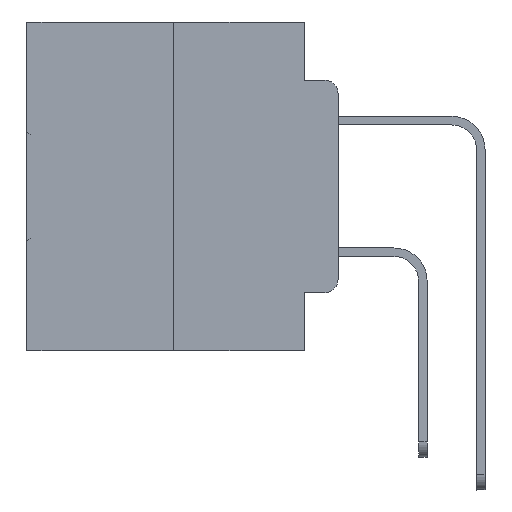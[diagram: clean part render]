
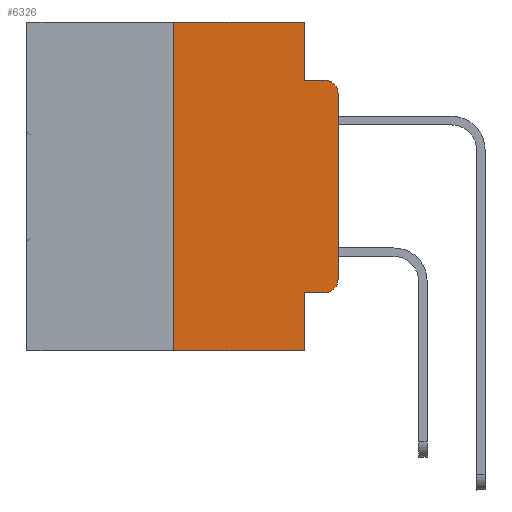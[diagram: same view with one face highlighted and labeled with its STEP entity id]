
A CAD part, left-side view. The second image highlights one B-rep face of the part: STEP entity #6326.
In plain terms, the highlighted planar face has unit normal (-1, 0, 0).
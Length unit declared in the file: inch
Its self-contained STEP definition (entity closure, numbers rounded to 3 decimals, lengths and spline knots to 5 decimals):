
#395 = CARTESIAN_POINT ( 'NONE',  ( 0., 0.051, -0.4115 ) ) ;
#605 = DIRECTION ( 'NONE',  ( 0., -1., 0. ) ) ;
#1468 = CARTESIAN_POINT ( 'NONE',  ( 0., 0.051, 0. ) ) ;
#1921 = CARTESIAN_POINT ( 'NONE',  ( 0., 0.473, 0. ) ) ;
#2920 = ORIENTED_EDGE ( 'NONE', *, *, #32133, .T. ) ;
#3748 = VERTEX_POINT ( 'NONE', #19978 ) ;
#4130 = ORIENTED_EDGE ( 'NONE', *, *, #6447, .T. ) ;
#4686 = FACE_OUTER_BOUND ( 'NONE', #32438, .T. ) ;
#4892 = LINE ( 'NONE', #25082, #20230 ) ;
#4902 = DIRECTION ( 'NONE',  ( 0., -1., 0. ) ) ;
#5497 = VECTOR ( 'NONE', #4902, 39.37008 ) ;
#5581 = VECTOR ( 'NONE', #5647, 39.37008 ) ;
#5647 = DIRECTION ( 'NONE',  ( 0., 0., 1. ) ) ;
#5932 = LINE ( 'NONE', #33000, #19574 ) ;
#6000 = EDGE_CURVE ( 'NONE', #9498, #12950, #12390, .T. ) ;
#6326 = ADVANCED_FACE ( 'NONE', ( #4686 ), #10875, .F. ) ;
#6447 = EDGE_CURVE ( 'NONE', #14063, #12950, #5932, .T. ) ;
#6592 = CARTESIAN_POINT ( 'NONE',  ( 0., 0.02, -0.1085 ) ) ;
#6674 = CARTESIAN_POINT ( 'NONE',  ( 0., 0.25, 0. ) ) ;
#6714 = VECTOR ( 'NONE', #28657, 39.37008 ) ;
#7404 = VECTOR ( 'NONE', #19513, 39.37008 ) ;
#7752 = AXIS2_PLACEMENT_3D ( 'NONE', #6592, #25586, #9332 ) ;
#7899 = EDGE_CURVE ( 'NONE', #23251, #21904, #24966, .T. ) ;
#8251 = DIRECTION ( 'NONE',  ( 0., 0., -1. ) ) ;
#9046 = EDGE_CURVE ( 'NONE', #9549, #3748, #10031, .T. ) ;
#9076 = ORIENTED_EDGE ( 'NONE', *, *, #33514, .F. ) ;
#9156 = CARTESIAN_POINT ( 'NONE',  ( 0., 0.051, -0.0885 ) ) ;
#9332 = DIRECTION ( 'NONE',  ( 0., 0., -1. ) ) ;
#9498 = VERTEX_POINT ( 'NONE', #395 ) ;
#9549 = VERTEX_POINT ( 'NONE', #22388 ) ;
#10031 = CIRCLE ( 'NONE', #12363, 0.02 ) ;
#10875 = PLANE ( 'NONE',  #23406 ) ;
#11300 = ORIENTED_EDGE ( 'NONE', *, *, #7899, .T. ) ;
#11799 = ORIENTED_EDGE ( 'NONE', *, *, #14082, .F. ) ;
#12113 = DIRECTION ( 'NONE',  ( -1., 0., 0. ) ) ;
#12363 = AXIS2_PLACEMENT_3D ( 'NONE', #28296, #12113, #30946 ) ;
#12390 = LINE ( 'NONE', #1468, #25947 ) ;
#12442 = DIRECTION ( 'NONE',  ( 0., 0., -1. ) ) ;
#12760 = LINE ( 'NONE', #1921, #5497 ) ;
#12950 = VERTEX_POINT ( 'NONE', #31614 ) ;
#13014 = EDGE_CURVE ( 'NONE', #30397, #27172, #12760, .T. ) ;
#13642 = VECTOR ( 'NONE', #22838, 39.37008 ) ;
#13964 = LINE ( 'NONE', #28777, #6714 ) ;
#14063 = VERTEX_POINT ( 'NONE', #20664 ) ;
#14082 = EDGE_CURVE ( 'NONE', #27130, #21904, #13964, .T. ) ;
#14679 = LINE ( 'NONE', #19395, #7404 ) ;
#15423 = ORIENTED_EDGE ( 'NONE', *, *, #6000, .F. ) ;
#15565 = EDGE_CURVE ( 'NONE', #27172, #27130, #4892, .T. ) ;
#16531 = CARTESIAN_POINT ( 'NONE',  ( 0., 0.25, 0. ) ) ;
#19069 = CARTESIAN_POINT ( 'NONE',  ( 0., 0.473, 0. ) ) ;
#19395 = CARTESIAN_POINT ( 'NONE',  ( 0., 0.051, -0.4115 ) ) ;
#19513 = DIRECTION ( 'NONE',  ( 0., -1., 0. ) ) ;
#19574 = VECTOR ( 'NONE', #605, 39.37008 ) ;
#19978 = CARTESIAN_POINT ( 'NONE',  ( 0., 0., -0.3915 ) ) ;
#20122 = CARTESIAN_POINT ( 'NONE',  ( 0., 0., 0. ) ) ;
#20230 = VECTOR ( 'NONE', #27755, 39.37008 ) ;
#20664 = CARTESIAN_POINT ( 'NONE',  ( 0., 0.25, -0.5 ) ) ;
#21017 = ORIENTED_EDGE ( 'NONE', *, *, #9046, .T. ) ;
#21904 = VERTEX_POINT ( 'NONE', #29065 ) ;
#22388 = CARTESIAN_POINT ( 'NONE',  ( 0., 0.02, -0.4115 ) ) ;
#22838 = DIRECTION ( 'NONE',  ( 0., 0., 1. ) ) ;
#23251 = VERTEX_POINT ( 'NONE', #29214 ) ;
#23406 = AXIS2_PLACEMENT_3D ( 'NONE', #19069, #24498, #8251 ) ;
#23587 = ORIENTED_EDGE ( 'NONE', *, *, #15565, .F. ) ;
#23698 = ORIENTED_EDGE ( 'NONE', *, *, #13014, .F. ) ;
#24498 = DIRECTION ( 'NONE',  ( 1., 0., 0. ) ) ;
#24714 = ORIENTED_EDGE ( 'NONE', *, *, #34378, .T. ) ;
#24966 = CIRCLE ( 'NONE', #7752, 0.02 ) ;
#25082 = CARTESIAN_POINT ( 'NONE',  ( 0., 0.051, 0. ) ) ;
#25586 = DIRECTION ( 'NONE',  ( -1., 0., 0. ) ) ;
#25947 = VECTOR ( 'NONE', #12442, 39.37008 ) ;
#27130 = VERTEX_POINT ( 'NONE', #9156 ) ;
#27172 = VERTEX_POINT ( 'NONE', #28337 ) ;
#27755 = DIRECTION ( 'NONE',  ( 0., 0., -1. ) ) ;
#28003 = LINE ( 'NONE', #20122, #13642 ) ;
#28296 = CARTESIAN_POINT ( 'NONE',  ( 0., 0.02, -0.3915 ) ) ;
#28337 = CARTESIAN_POINT ( 'NONE',  ( 0., 0.051, 0. ) ) ;
#28657 = DIRECTION ( 'NONE',  ( 0., -1., 0. ) ) ;
#28777 = CARTESIAN_POINT ( 'NONE',  ( 0., 0.051, -0.0885 ) ) ;
#29065 = CARTESIAN_POINT ( 'NONE',  ( 0., 0.02, -0.0885 ) ) ;
#29214 = CARTESIAN_POINT ( 'NONE',  ( 0., 0., -0.1085 ) ) ;
#30397 = VERTEX_POINT ( 'NONE', #6674 ) ;
#30946 = DIRECTION ( 'NONE',  ( 0., 0., -1. ) ) ;
#31614 = CARTESIAN_POINT ( 'NONE',  ( 0., 0.051, -0.5 ) ) ;
#32133 = EDGE_CURVE ( 'NONE', #9498, #9549, #14679, .T. ) ;
#32438 = EDGE_LOOP ( 'NONE', ( #24714, #11300, #11799, #23587, #23698, #9076, #4130, #15423, #2920, #21017 ) ) ;
#33000 = CARTESIAN_POINT ( 'NONE',  ( 0., 0.473, -0.5 ) ) ;
#33514 = EDGE_CURVE ( 'NONE', #14063, #30397, #34301, .T. ) ;
#34301 = LINE ( 'NONE', #16531, #5581 ) ;
#34378 = EDGE_CURVE ( 'NONE', #3748, #23251, #28003, .T. ) ;
